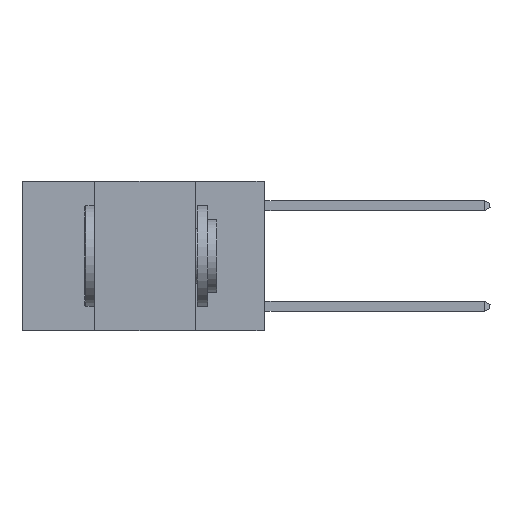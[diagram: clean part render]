
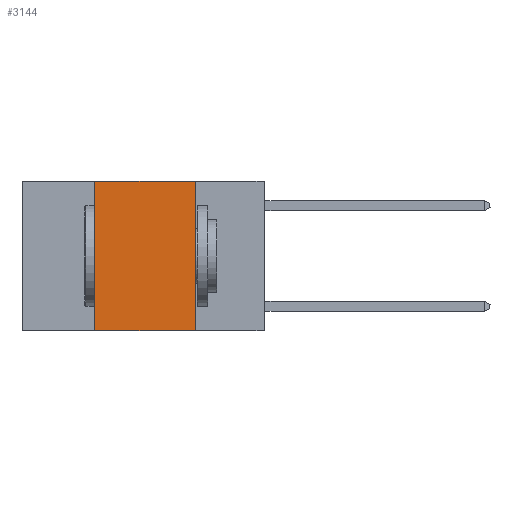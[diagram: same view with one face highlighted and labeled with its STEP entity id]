
A CAD part, left-side view. The second image highlights one B-rep face of the part: STEP entity #3144.
In plain terms, the highlighted planar face has unit normal (-1, 0, 0).
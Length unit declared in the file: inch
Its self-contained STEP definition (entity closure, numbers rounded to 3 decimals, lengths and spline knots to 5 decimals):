
#101 = LINE ( 'NONE', #8100, #10339 ) ;
#166 = ORIENTED_EDGE ( 'NONE', *, *, #8587, .T. ) ;
#572 = EDGE_CURVE ( 'NONE', #6382, #10947, #13107, .T. ) ;
#781 = CARTESIAN_POINT ( 'NONE',  ( 0., 0.17, -0.37 ) ) ;
#927 = VECTOR ( 'NONE', #17255, 39.37008 ) ;
#1458 = ORIENTED_EDGE ( 'NONE', *, *, #13155, .F. ) ;
#3131 = CARTESIAN_POINT ( 'NONE',  ( 0., 0.42, -0.37 ) ) ;
#3144 = ADVANCED_FACE ( 'NONE', ( #17111 ), #16934, .F. ) ;
#3285 = DIRECTION ( 'NONE',  ( 1., 0., 0. ) ) ;
#3369 = VECTOR ( 'NONE', #12444, 39.37008 ) ;
#4336 = DIRECTION ( 'NONE',  ( 0., -1., 0. ) ) ;
#4422 = DIRECTION ( 'NONE',  ( 0., 0., 1. ) ) ;
#4537 = DIRECTION ( 'NONE',  ( 0., 0., -1. ) ) ;
#5339 = EDGE_CURVE ( 'NONE', #12481, #7042, #101, .T. ) ;
#5702 = CARTESIAN_POINT ( 'NONE',  ( 0., 0.6, -0.37 ) ) ;
#6289 = CARTESIAN_POINT ( 'NONE',  ( 0., 0.42, 0. ) ) ;
#6382 = VERTEX_POINT ( 'NONE', #14066 ) ;
#7042 = VERTEX_POINT ( 'NONE', #6289 ) ;
#8100 = CARTESIAN_POINT ( 'NONE',  ( 0., 0.42, 0. ) ) ;
#8587 = EDGE_CURVE ( 'NONE', #12481, #10947, #13811, .T. ) ;
#8918 = CARTESIAN_POINT ( 'NONE',  ( 0., 0.6, 0. ) ) ;
#8984 = CARTESIAN_POINT ( 'NONE',  ( 0., 0.17, 0. ) ) ;
#10339 = VECTOR ( 'NONE', #4422, 39.37008 ) ;
#10947 = VERTEX_POINT ( 'NONE', #781 ) ;
#11137 = CARTESIAN_POINT ( 'NONE',  ( 0., 0.6, 0. ) ) ;
#11678 = AXIS2_PLACEMENT_3D ( 'NONE', #8918, #3285, #4537 ) ;
#12444 = DIRECTION ( 'NONE',  ( 0., -1., 0. ) ) ;
#12481 = VERTEX_POINT ( 'NONE', #3131 ) ;
#12894 = VECTOR ( 'NONE', #4336, 39.37008 ) ;
#13107 = LINE ( 'NONE', #8984, #927 ) ;
#13155 = EDGE_CURVE ( 'NONE', #7042, #6382, #15292, .T. ) ;
#13811 = LINE ( 'NONE', #5702, #3369 ) ;
#14066 = CARTESIAN_POINT ( 'NONE',  ( 0., 0.17, 0. ) ) ;
#14364 = ORIENTED_EDGE ( 'NONE', *, *, #572, .F. ) ;
#14643 = ORIENTED_EDGE ( 'NONE', *, *, #5339, .F. ) ;
#15292 = LINE ( 'NONE', #11137, #12894 ) ;
#16245 = EDGE_LOOP ( 'NONE', ( #14364, #1458, #14643, #166 ) ) ;
#16934 = PLANE ( 'NONE',  #11678 ) ;
#17111 = FACE_OUTER_BOUND ( 'NONE', #16245, .T. ) ;
#17255 = DIRECTION ( 'NONE',  ( 0., 0., -1. ) ) ;
